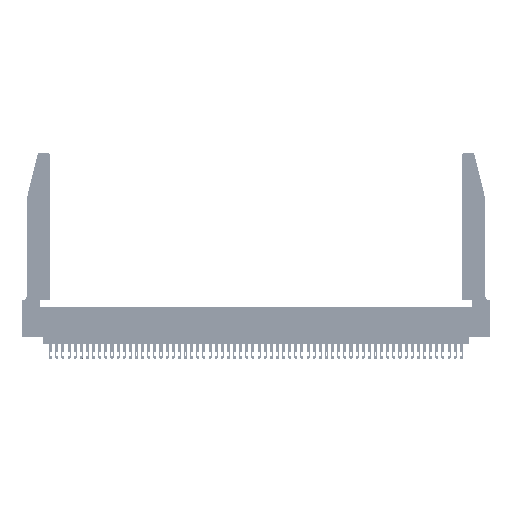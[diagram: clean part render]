
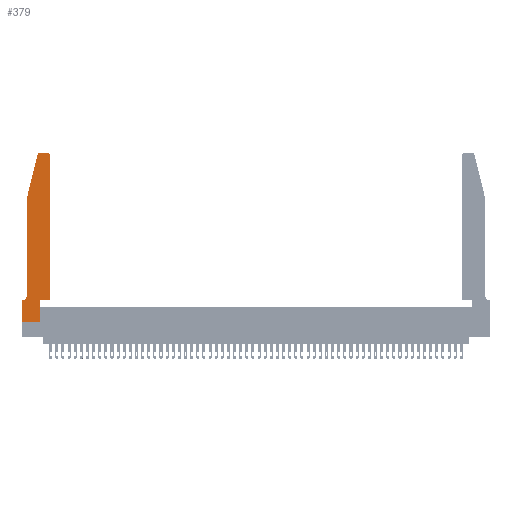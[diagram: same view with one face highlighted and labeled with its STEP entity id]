
A CAD part, top view. The second image highlights one B-rep face of the part: STEP entity #379.
In plain terms, the highlighted planar face has unit normal (0, 0, 1).
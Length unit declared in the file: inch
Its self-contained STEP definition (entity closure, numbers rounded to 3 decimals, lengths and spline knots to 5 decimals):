
#379 = ADVANCED_FACE ( 'NONE', ( #2671 ), #44123, .T. ) ;
#827 = AXIS2_PLACEMENT_3D ( 'NONE', #50659, #41787, #42166 ) ;
#1264 = CARTESIAN_POINT ( 'NONE',  ( 0.4505, 0.35, 0.37 ) ) ;
#1436 = CARTESIAN_POINT ( 'NONE',  ( 0., 0., 0.37 ) ) ;
#1522 = DIRECTION ( 'NONE',  ( 0., 0., 1. ) ) ;
#1914 = VERTEX_POINT ( 'NONE', #2678 ) ;
#2613 = ORIENTED_EDGE ( 'NONE', *, *, #15474, .T. ) ;
#2671 = FACE_OUTER_BOUND ( 'NONE', #7676, .T. ) ;
#2678 = CARTESIAN_POINT ( 'NONE',  ( 0., 0.35, 0.37 ) ) ;
#2962 = VECTOR ( 'NONE', #53322, 39.37008 ) ;
#3483 = CARTESIAN_POINT ( 'NONE',  ( 0., 0., 0.37 ) ) ;
#3556 = CARTESIAN_POINT ( 'NONE',  ( 0.4505, 2.72, 0.37 ) ) ;
#4896 = DIRECTION ( 'NONE',  ( 0., 0., -1. ) ) ;
#6172 = VERTEX_POINT ( 'NONE', #3556 ) ;
#7548 = EDGE_CURVE ( 'NONE', #19761, #6172, #12188, .T. ) ;
#7676 = EDGE_LOOP ( 'NONE', ( #2613, #22800, #22660, #28422, #31689, #44755, #39328, #41418, #22693, #52220, #10006, #39567 ) ) ;
#9479 = VERTEX_POINT ( 'NONE', #24606 ) ;
#10006 = ORIENTED_EDGE ( 'NONE', *, *, #7548, .T. ) ;
#10646 = AXIS2_PLACEMENT_3D ( 'NONE', #14417, #39826, #14233 ) ;
#11182 = EDGE_CURVE ( 'NONE', #6172, #9479, #12675, .T. ) ;
#11524 = LINE ( 'NONE', #26434, #35910 ) ;
#11702 = VERTEX_POINT ( 'NONE', #43133 ) ;
#11962 = EDGE_CURVE ( 'NONE', #21605, #19761, #13209, .T. ) ;
#12188 = LINE ( 'NONE', #13387, #39198 ) ;
#12240 = LINE ( 'NONE', #3483, #2962 ) ;
#12675 = CIRCLE ( 'NONE', #10646, 0.03 ) ;
#13209 = LINE ( 'NONE', #40528, #35614 ) ;
#13387 = CARTESIAN_POINT ( 'NONE',  ( 0.4505, 0.35, 0.37 ) ) ;
#13406 = CIRCLE ( 'NONE', #827, 0.03 ) ;
#13933 = CARTESIAN_POINT ( 'NONE',  ( 0.2605, 2.75, 0.37 ) ) ;
#14200 = LINE ( 'NONE', #13933, #16142 ) ;
#14233 = DIRECTION ( 'NONE',  ( 1., 0., 0. ) ) ;
#14417 = CARTESIAN_POINT ( 'NONE',  ( 0.4205, 2.72, 0.37 ) ) ;
#14504 = EDGE_CURVE ( 'NONE', #1914, #35993, #12240, .T. ) ;
#14649 = CARTESIAN_POINT ( 'NONE',  ( 0., 0.35, 0.37 ) ) ;
#15474 = EDGE_CURVE ( 'NONE', #9479, #11702, #14200, .T. ) ;
#15994 = EDGE_CURVE ( 'NONE', #28030, #21605, #11524, .T. ) ;
#16142 = VECTOR ( 'NONE', #17424, 39.37008 ) ;
#17269 = LINE ( 'NONE', #17799, #22582 ) ;
#17424 = DIRECTION ( 'NONE',  ( -1., 0., 0. ) ) ;
#17799 = CARTESIAN_POINT ( 'NONE',  ( 0.0755, 2., 0.37 ) ) ;
#18360 = DIRECTION ( 'NONE',  ( 0., -1., 0. ) ) ;
#19761 = VERTEX_POINT ( 'NONE', #1264 ) ;
#19940 = DIRECTION ( 'NONE',  ( 1., 0., 0. ) ) ;
#20079 = LINE ( 'NONE', #27425, #33273 ) ;
#20132 = AXIS2_PLACEMENT_3D ( 'NONE', #43057, #4896, #21722 ) ;
#20692 = EDGE_CURVE ( 'NONE', #37054, #41980, #20961, .T. ) ;
#20961 = CIRCLE ( 'NONE', #20132, 0.07 ) ;
#21605 = VERTEX_POINT ( 'NONE', #27907 ) ;
#21722 = DIRECTION ( 'NONE',  ( -1., 0., 0. ) ) ;
#22582 = VECTOR ( 'NONE', #18360, 39.37008 ) ;
#22660 = ORIENTED_EDGE ( 'NONE', *, *, #26451, .T. ) ;
#22693 = ORIENTED_EDGE ( 'NONE', *, *, #15994, .T. ) ;
#22800 = ORIENTED_EDGE ( 'NONE', *, *, #32484, .T. ) ;
#24606 = CARTESIAN_POINT ( 'NONE',  ( 0.4205, 2.75, 0.37 ) ) ;
#26434 = CARTESIAN_POINT ( 'NONE',  ( 0.2865, 0.35, 0.37 ) ) ;
#26451 = EDGE_CURVE ( 'NONE', #26786, #37121, #46059, .T. ) ;
#26786 = VERTEX_POINT ( 'NONE', #33978 ) ;
#27425 = CARTESIAN_POINT ( 'NONE',  ( 0.0755, 0.35, 0.37 ) ) ;
#27732 = DIRECTION ( 'NONE',  ( -0.239, -0.971, 0. ) ) ;
#27907 = CARTESIAN_POINT ( 'NONE',  ( 0.2865, 0.35, 0.37 ) ) ;
#28030 = VERTEX_POINT ( 'NONE', #37128 ) ;
#28422 = ORIENTED_EDGE ( 'NONE', *, *, #47193, .T. ) ;
#30904 = DIRECTION ( 'NONE',  ( 1., 0., 0. ) ) ;
#31689 = ORIENTED_EDGE ( 'NONE', *, *, #20692, .T. ) ;
#31900 = DIRECTION ( 'NONE',  ( 1., 0., 0. ) ) ;
#32224 = DIRECTION ( 'NONE',  ( -1., 0., 0. ) ) ;
#32484 = EDGE_CURVE ( 'NONE', #11702, #26786, #13406, .T. ) ;
#32810 = CARTESIAN_POINT ( 'NONE',  ( 0.0755, 0.42, 0.37 ) ) ;
#33273 = VECTOR ( 'NONE', #32224, 39.37008 ) ;
#33978 = CARTESIAN_POINT ( 'NONE',  ( 0.25487, 2.72718, 0.37 ) ) ;
#35614 = VECTOR ( 'NONE', #19940, 39.37008 ) ;
#35910 = VECTOR ( 'NONE', #47767, 39.37008 ) ;
#35993 = VERTEX_POINT ( 'NONE', #37261 ) ;
#36883 = EDGE_CURVE ( 'NONE', #35993, #28030, #44764, .T. ) ;
#37054 = VERTEX_POINT ( 'NONE', #32810 ) ;
#37121 = VERTEX_POINT ( 'NONE', #49382 ) ;
#37128 = CARTESIAN_POINT ( 'NONE',  ( 0.2865, 0., 0.37 ) ) ;
#37261 = CARTESIAN_POINT ( 'NONE',  ( 0., 0., 0.37 ) ) ;
#39198 = VECTOR ( 'NONE', #51371, 39.37008 ) ;
#39328 = ORIENTED_EDGE ( 'NONE', *, *, #14504, .T. ) ;
#39567 = ORIENTED_EDGE ( 'NONE', *, *, #11182, .T. ) ;
#39826 = DIRECTION ( 'NONE',  ( 0., 0., 1. ) ) ;
#40528 = CARTESIAN_POINT ( 'NONE',  ( 0.4505, 0.35, 0.37 ) ) ;
#41418 = ORIENTED_EDGE ( 'NONE', *, *, #36883, .T. ) ;
#41453 = VECTOR ( 'NONE', #27732, 39.37008 ) ;
#41787 = DIRECTION ( 'NONE',  ( 0., 0., 1. ) ) ;
#41980 = VERTEX_POINT ( 'NONE', #42397 ) ;
#42104 = VECTOR ( 'NONE', #31900, 39.37008 ) ;
#42166 = DIRECTION ( 'NONE',  ( 1., 0., 0. ) ) ;
#42397 = CARTESIAN_POINT ( 'NONE',  ( 0.0055, 0.35, 0.37 ) ) ;
#42496 = AXIS2_PLACEMENT_3D ( 'NONE', #14649, #1522, #30904 ) ;
#43057 = CARTESIAN_POINT ( 'NONE',  ( 0.0055, 0.42, 0.37 ) ) ;
#43133 = CARTESIAN_POINT ( 'NONE',  ( 0.284, 2.75, 0.37 ) ) ;
#44123 = PLANE ( 'NONE',  #42496 ) ;
#44755 = ORIENTED_EDGE ( 'NONE', *, *, #52441, .T. ) ;
#44764 = LINE ( 'NONE', #1436, #42104 ) ;
#46059 = LINE ( 'NONE', #52440, #41453 ) ;
#47193 = EDGE_CURVE ( 'NONE', #37121, #37054, #17269, .T. ) ;
#47767 = DIRECTION ( 'NONE',  ( 0., 1., 0. ) ) ;
#49382 = CARTESIAN_POINT ( 'NONE',  ( 0.0755, 2., 0.37 ) ) ;
#50659 = CARTESIAN_POINT ( 'NONE',  ( 0.284, 2.72, 0.37 ) ) ;
#51371 = DIRECTION ( 'NONE',  ( 0., 1., 0. ) ) ;
#52220 = ORIENTED_EDGE ( 'NONE', *, *, #11962, .T. ) ;
#52440 = CARTESIAN_POINT ( 'NONE',  ( 0.0755, 2., 0.37 ) ) ;
#52441 = EDGE_CURVE ( 'NONE', #41980, #1914, #20079, .T. ) ;
#53322 = DIRECTION ( 'NONE',  ( 0., -1., 0. ) ) ;
